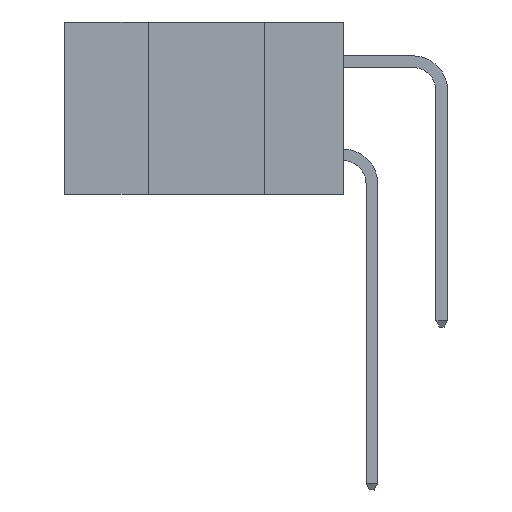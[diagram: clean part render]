
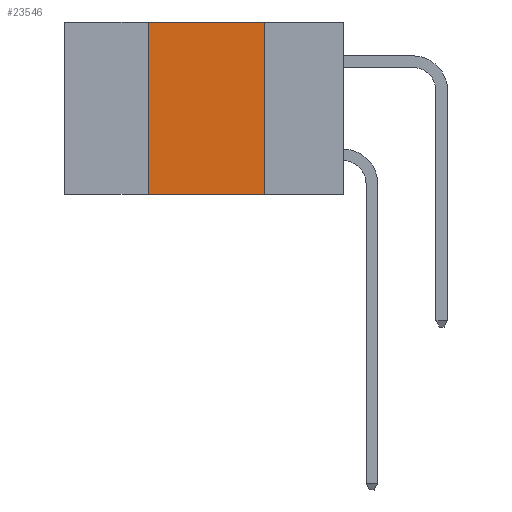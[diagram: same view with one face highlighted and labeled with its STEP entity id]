
A CAD part, left-side view. The second image highlights one B-rep face of the part: STEP entity #23546.
In plain terms, the highlighted planar face has unit normal (-1, 0, 0).
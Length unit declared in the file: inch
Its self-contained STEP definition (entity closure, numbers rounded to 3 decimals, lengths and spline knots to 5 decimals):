
#71 = DIRECTION ( 'NONE',  ( 0., -1., 0. ) ) ;
#573 = VECTOR ( 'NONE', #9340, 39.37008 ) ;
#800 = CARTESIAN_POINT ( 'NONE',  ( 0., 0.6, -0.37 ) ) ;
#2299 = LINE ( 'NONE', #13582, #6449 ) ;
#4656 = ORIENTED_EDGE ( 'NONE', *, *, #25189, .F. ) ;
#5432 = VECTOR ( 'NONE', #12588, 39.37008 ) ;
#5661 = CARTESIAN_POINT ( 'NONE',  ( 0., 0.6, 0. ) ) ;
#5810 = EDGE_CURVE ( 'NONE', #23243, #32658, #7122, .T. ) ;
#6449 = VECTOR ( 'NONE', #71, 39.37008 ) ;
#7122 = LINE ( 'NONE', #34146, #5432 ) ;
#8374 = VERTEX_POINT ( 'NONE', #15504 ) ;
#9340 = DIRECTION ( 'NONE',  ( 0., 0., -1. ) ) ;
#10647 = ORIENTED_EDGE ( 'NONE', *, *, #5810, .F. ) ;
#12588 = DIRECTION ( 'NONE',  ( 0., 0., 1. ) ) ;
#13582 = CARTESIAN_POINT ( 'NONE',  ( 0., 0.6, 0. ) ) ;
#13963 = DIRECTION ( 'NONE',  ( 0., -1., 0. ) ) ;
#15504 = CARTESIAN_POINT ( 'NONE',  ( 0., 0.17, -0.37 ) ) ;
#17081 = EDGE_CURVE ( 'NONE', #19618, #8374, #21007, .T. ) ;
#18360 = CARTESIAN_POINT ( 'NONE',  ( 0., 0.17, 0. ) ) ;
#19548 = ORIENTED_EDGE ( 'NONE', *, *, #17081, .F. ) ;
#19618 = VERTEX_POINT ( 'NONE', #18360 ) ;
#20414 = VECTOR ( 'NONE', #13963, 39.37008 ) ;
#21007 = LINE ( 'NONE', #33492, #573 ) ;
#21198 = DIRECTION ( 'NONE',  ( 1., 0., 0. ) ) ;
#21654 = PLANE ( 'NONE',  #34408 ) ;
#22301 = EDGE_CURVE ( 'NONE', #23243, #8374, #25388, .T. ) ;
#22306 = EDGE_LOOP ( 'NONE', ( #19548, #4656, #10647, #24314 ) ) ;
#23243 = VERTEX_POINT ( 'NONE', #29621 ) ;
#23546 = ADVANCED_FACE ( 'NONE', ( #32046 ), #21654, .F. ) ;
#24305 = DIRECTION ( 'NONE',  ( 0., 0., -1. ) ) ;
#24314 = ORIENTED_EDGE ( 'NONE', *, *, #22301, .T. ) ;
#25189 = EDGE_CURVE ( 'NONE', #32658, #19618, #2299, .T. ) ;
#25388 = LINE ( 'NONE', #800, #20414 ) ;
#29621 = CARTESIAN_POINT ( 'NONE',  ( 0., 0.42, -0.37 ) ) ;
#31437 = CARTESIAN_POINT ( 'NONE',  ( 0., 0.42, 0. ) ) ;
#32046 = FACE_OUTER_BOUND ( 'NONE', #22306, .T. ) ;
#32658 = VERTEX_POINT ( 'NONE', #31437 ) ;
#33492 = CARTESIAN_POINT ( 'NONE',  ( 0., 0.17, 0. ) ) ;
#34146 = CARTESIAN_POINT ( 'NONE',  ( 0., 0.42, 0. ) ) ;
#34408 = AXIS2_PLACEMENT_3D ( 'NONE', #5661, #21198, #24305 ) ;
